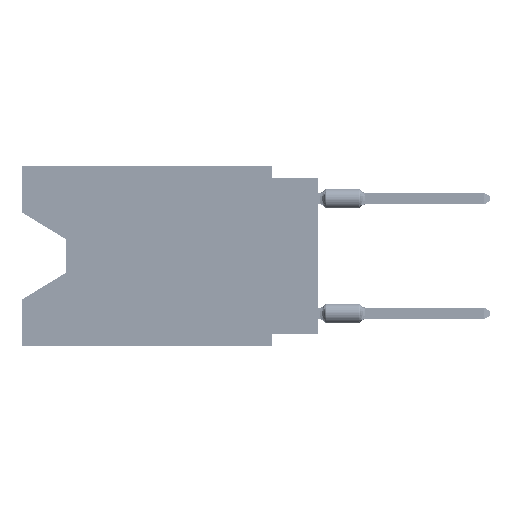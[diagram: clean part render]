
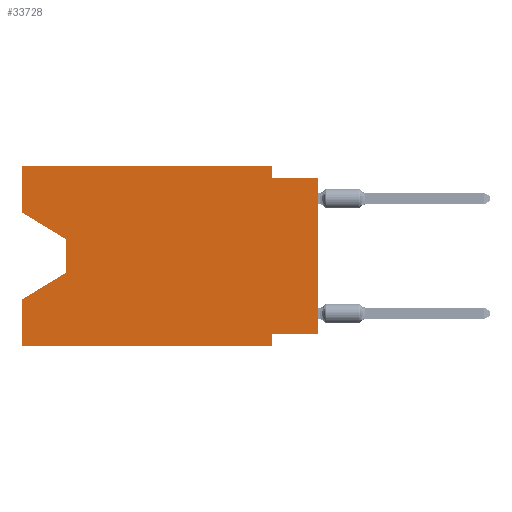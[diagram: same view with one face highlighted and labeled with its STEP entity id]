
A CAD part, left-side view. The second image highlights one B-rep face of the part: STEP entity #33728.
In plain terms, the highlighted planar face has unit normal (-1, 0, 0).
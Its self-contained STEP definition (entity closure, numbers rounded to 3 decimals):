
#2477 = CARTESIAN_POINT ( 'NONE',  ( 0., 13.97, -5.893 ) ) ;
#2674 = DIRECTION ( 'NONE',  ( 1., 0., 0. ) ) ;
#3321 = LINE ( 'NONE', #48953, #67774 ) ;
#3670 = LINE ( 'NONE', #30594, #61790 ) ;
#6033 = EDGE_CURVE ( 'NONE', #56858, #46027, #39147, .T. ) ;
#6179 = CARTESIAN_POINT ( 'NONE',  ( 0., 2.54, 0. ) ) ;
#6891 = DIRECTION ( 'NONE',  ( 0., -1., 0. ) ) ;
#7014 = VERTEX_POINT ( 'NONE', #34129 ) ;
#8471 = CARTESIAN_POINT ( 'NONE',  ( 0., 0., -0.635 ) ) ;
#10037 = CARTESIAN_POINT ( 'NONE',  ( 0., 0., -9.271 ) ) ;
#10644 = CARTESIAN_POINT ( 'NONE',  ( 0., 16.383, -9.906 ) ) ;
#11010 = CARTESIAN_POINT ( 'NONE',  ( 0., 0., -9.271 ) ) ;
#13015 = ORIENTED_EDGE ( 'NONE', *, *, #80015, .F. ) ;
#13874 = CARTESIAN_POINT ( 'NONE',  ( 0., 16.383, 0. ) ) ;
#14630 = VECTOR ( 'NONE', #34989, 1000. ) ;
#16257 = EDGE_CURVE ( 'NONE', #46027, #44281, #17060, .T. ) ;
#17060 = LINE ( 'NONE', #44858, #75453 ) ;
#17128 = DIRECTION ( 'NONE',  ( 0., 0., 1. ) ) ;
#17343 = CARTESIAN_POINT ( 'NONE',  ( 0., 0., 0. ) ) ;
#18025 = CARTESIAN_POINT ( 'NONE',  ( 0., 16.383, -2.546 ) ) ;
#19859 = EDGE_CURVE ( 'NONE', #75841, #7014, #3670, .T. ) ;
#20094 = LINE ( 'NONE', #47048, #26201 ) ;
#21052 = CARTESIAN_POINT ( 'NONE',  ( 0., 16.383, -9.906 ) ) ;
#23057 = CARTESIAN_POINT ( 'NONE',  ( 0., 16.383, 0. ) ) ;
#23995 = EDGE_CURVE ( 'NONE', #75841, #44281, #34115, .T. ) ;
#24288 = EDGE_CURVE ( 'NONE', #28060, #57292, #20094, .T. ) ;
#25629 = DIRECTION ( 'NONE',  ( 0., -0.855, -0.519 ) ) ;
#26201 = VECTOR ( 'NONE', #67030, 1000. ) ;
#26668 = VERTEX_POINT ( 'NONE', #2477 ) ;
#26887 = ORIENTED_EDGE ( 'NONE', *, *, #6033, .F. ) ;
#27844 = EDGE_CURVE ( 'NONE', #26668, #7014, #42750, .T. ) ;
#28060 = VERTEX_POINT ( 'NONE', #6179 ) ;
#30594 = CARTESIAN_POINT ( 'NONE',  ( 0., 16.383, 0. ) ) ;
#33728 = ADVANCED_FACE ( 'NONE', ( #56090 ), #82584, .F. ) ;
#34115 = LINE ( 'NONE', #21052, #71940 ) ;
#34129 = CARTESIAN_POINT ( 'NONE',  ( 0., 16.383, -7.36 ) ) ;
#34989 = DIRECTION ( 'NONE',  ( 0., -1., 0. ) ) ;
#35115 = VERTEX_POINT ( 'NONE', #70864 ) ;
#35345 = VERTEX_POINT ( 'NONE', #18025 ) ;
#35932 = DIRECTION ( 'NONE',  ( 0., 0., 1. ) ) ;
#36066 = LINE ( 'NONE', #17343, #39210 ) ;
#36147 = VECTOR ( 'NONE', #42319, 1000. ) ;
#37420 = LINE ( 'NONE', #84731, #64772 ) ;
#39147 = LINE ( 'NONE', #11010, #80025 ) ;
#39210 = VECTOR ( 'NONE', #50370, 1000. ) ;
#40538 = VECTOR ( 'NONE', #6891, 1000. ) ;
#41070 = DIRECTION ( 'NONE',  ( 0., -1., 0. ) ) ;
#41111 = EDGE_CURVE ( 'NONE', #35345, #35115, #77360, .T. ) ;
#42319 = DIRECTION ( 'NONE',  ( 0., 0.855, -0.519 ) ) ;
#42750 = LINE ( 'NONE', #69251, #36147 ) ;
#42944 = ORIENTED_EDGE ( 'NONE', *, *, #57058, .T. ) ;
#43568 = DIRECTION ( 'NONE',  ( 0., 0., -1. ) ) ;
#43992 = EDGE_CURVE ( 'NONE', #35345, #45367, #3321, .T. ) ;
#44281 = VERTEX_POINT ( 'NONE', #72262 ) ;
#44858 = CARTESIAN_POINT ( 'NONE',  ( 0., 2.54, -9.906 ) ) ;
#44870 = ORIENTED_EDGE ( 'NONE', *, *, #23995, .T. ) ;
#45367 = VERTEX_POINT ( 'NONE', #82828 ) ;
#45962 = ORIENTED_EDGE ( 'NONE', *, *, #41111, .T. ) ;
#46027 = VERTEX_POINT ( 'NONE', #67049 ) ;
#47048 = CARTESIAN_POINT ( 'NONE',  ( 0., 2.54, 0. ) ) ;
#47351 = LINE ( 'NONE', #13874, #40538 ) ;
#48003 = ORIENTED_EDGE ( 'NONE', *, *, #65728, .T. ) ;
#48953 = CARTESIAN_POINT ( 'NONE',  ( 0., 16.383, 0. ) ) ;
#50370 = DIRECTION ( 'NONE',  ( 0., 0., 1. ) ) ;
#50381 = ORIENTED_EDGE ( 'NONE', *, *, #43992, .F. ) ;
#50565 = ORIENTED_EDGE ( 'NONE', *, *, #16257, .F. ) ;
#51007 = VECTOR ( 'NONE', #25629, 1000. ) ;
#55249 = DIRECTION ( 'NONE',  ( 0., 0., -1. ) ) ;
#56090 = FACE_OUTER_BOUND ( 'NONE', #59819, .T. ) ;
#56858 = VERTEX_POINT ( 'NONE', #10037 ) ;
#57058 = EDGE_CURVE ( 'NONE', #35115, #26668, #37420, .T. ) ;
#57292 = VERTEX_POINT ( 'NONE', #75563 ) ;
#58393 = ORIENTED_EDGE ( 'NONE', *, *, #78088, .F. ) ;
#59819 = EDGE_LOOP ( 'NONE', ( #45962, #42944, #70687, #83296, #44870, #50565, #26887, #48003, #13015, #70888, #58393, #50381 ) ) ;
#61790 = VECTOR ( 'NONE', #17128, 1000. ) ;
#64238 = AXIS2_PLACEMENT_3D ( 'NONE', #23057, #2674, #55249 ) ;
#64772 = VECTOR ( 'NONE', #83866, 1000. ) ;
#65728 = EDGE_CURVE ( 'NONE', #56858, #73770, #36066, .T. ) ;
#65796 = CARTESIAN_POINT ( 'NONE',  ( 0., 0., -0.635 ) ) ;
#67030 = DIRECTION ( 'NONE',  ( 0., 0., -1. ) ) ;
#67049 = CARTESIAN_POINT ( 'NONE',  ( 0., 2.54, -9.271 ) ) ;
#67774 = VECTOR ( 'NONE', #35932, 1000. ) ;
#68010 = LINE ( 'NONE', #8471, #14630 ) ;
#69251 = CARTESIAN_POINT ( 'NONE',  ( 0., 13.97, -5.893 ) ) ;
#70687 = ORIENTED_EDGE ( 'NONE', *, *, #27844, .T. ) ;
#70864 = CARTESIAN_POINT ( 'NONE',  ( 0., 13.97, -4.013 ) ) ;
#70888 = ORIENTED_EDGE ( 'NONE', *, *, #24288, .F. ) ;
#71940 = VECTOR ( 'NONE', #41070, 1000. ) ;
#72262 = CARTESIAN_POINT ( 'NONE',  ( 0., 2.54, -9.906 ) ) ;
#73770 = VERTEX_POINT ( 'NONE', #65796 ) ;
#75453 = VECTOR ( 'NONE', #43568, 1000. ) ;
#75563 = CARTESIAN_POINT ( 'NONE',  ( 0., 2.54, -0.635 ) ) ;
#75841 = VERTEX_POINT ( 'NONE', #10644 ) ;
#77360 = LINE ( 'NONE', #85151, #51007 ) ;
#78088 = EDGE_CURVE ( 'NONE', #45367, #28060, #47351, .T. ) ;
#79076 = DIRECTION ( 'NONE',  ( 0., 1., 0. ) ) ;
#80015 = EDGE_CURVE ( 'NONE', #57292, #73770, #68010, .T. ) ;
#80025 = VECTOR ( 'NONE', #79076, 1000. ) ;
#82584 = PLANE ( 'NONE',  #64238 ) ;
#82828 = CARTESIAN_POINT ( 'NONE',  ( 0., 16.383, 0. ) ) ;
#83296 = ORIENTED_EDGE ( 'NONE', *, *, #19859, .F. ) ;
#83866 = DIRECTION ( 'NONE',  ( 0., 0., -1. ) ) ;
#84731 = CARTESIAN_POINT ( 'NONE',  ( 0., 13.97, -4.013 ) ) ;
#85151 = CARTESIAN_POINT ( 'NONE',  ( 0., 16.383, -2.546 ) ) ;
